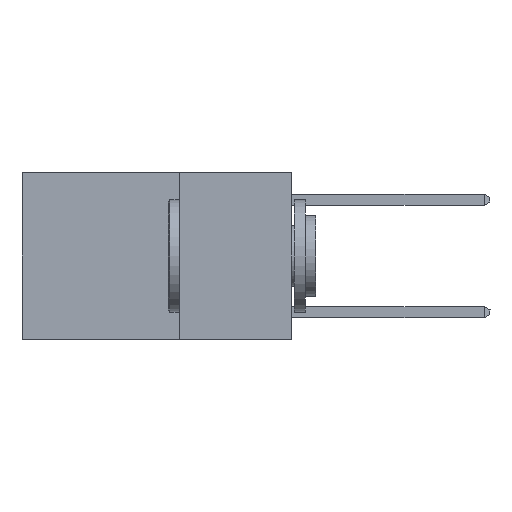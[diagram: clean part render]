
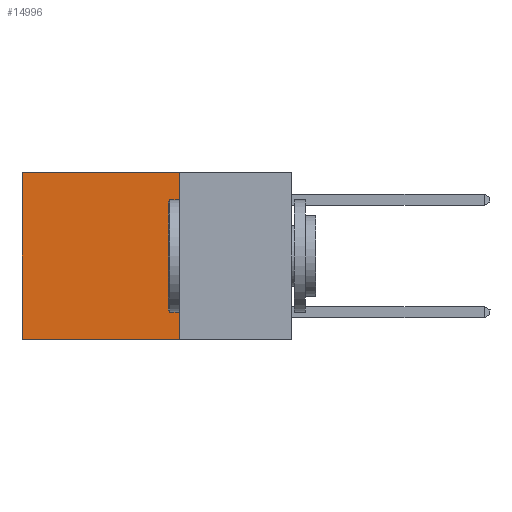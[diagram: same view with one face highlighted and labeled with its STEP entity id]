
A CAD part, left-side view. The second image highlights one B-rep face of the part: STEP entity #14996.
In plain terms, the highlighted planar face has unit normal (-1, 0, 0).
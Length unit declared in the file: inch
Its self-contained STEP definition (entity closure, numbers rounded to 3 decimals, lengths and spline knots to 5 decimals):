
#181 = AXIS2_PLACEMENT_3D ( 'NONE', #5114, #21425, #7490 ) ;
#1319 = EDGE_LOOP ( 'NONE', ( #19151, #2200, #12955, #26617 ) ) ;
#2108 = DIRECTION ( 'NONE',  ( 0., 0., -1. ) ) ;
#2200 = ORIENTED_EDGE ( 'NONE', *, *, #19887, .F. ) ;
#2207 = VECTOR ( 'NONE', #11178, 39.37008 ) ;
#2541 = VERTEX_POINT ( 'NONE', #19791 ) ;
#3071 = VERTEX_POINT ( 'NONE', #17153 ) ;
#5114 = CARTESIAN_POINT ( 'NONE',  ( 0.2625, 0.25, 0. ) ) ;
#6052 = CARTESIAN_POINT ( 'NONE',  ( 0.2625, 0.25, -0.37 ) ) ;
#7490 = DIRECTION ( 'NONE',  ( 0., 0., -1. ) ) ;
#9042 = EDGE_CURVE ( 'NONE', #3071, #2541, #26796, .T. ) ;
#9357 = EDGE_CURVE ( 'NONE', #2541, #21891, #18449, .T. ) ;
#10649 = DIRECTION ( 'NONE',  ( 0., 1., 0. ) ) ;
#11178 = DIRECTION ( 'NONE',  ( 0., 1., 0. ) ) ;
#12040 = LINE ( 'NONE', #29497, #29207 ) ;
#12274 = CARTESIAN_POINT ( 'NONE',  ( 0.2625, 0.6, 0. ) ) ;
#12849 = VERTEX_POINT ( 'NONE', #6052 ) ;
#12955 = ORIENTED_EDGE ( 'NONE', *, *, #15493, .F. ) ;
#12991 = VECTOR ( 'NONE', #14617, 39.37008 ) ;
#14617 = DIRECTION ( 'NONE',  ( 0., 0., -1. ) ) ;
#14996 = ADVANCED_FACE ( 'NONE', ( #18600 ), #27887, .F. ) ;
#15493 = EDGE_CURVE ( 'NONE', #3071, #12849, #12040, .T. ) ;
#17153 = CARTESIAN_POINT ( 'NONE',  ( 0.2625, 0.25, 0. ) ) ;
#18449 = LINE ( 'NONE', #12274, #12991 ) ;
#18600 = FACE_OUTER_BOUND ( 'NONE', #1319, .T. ) ;
#19151 = ORIENTED_EDGE ( 'NONE', *, *, #9357, .T. ) ;
#19791 = CARTESIAN_POINT ( 'NONE',  ( 0.2625, 0.6, 0. ) ) ;
#19859 = VECTOR ( 'NONE', #10649, 39.37008 ) ;
#19887 = EDGE_CURVE ( 'NONE', #12849, #21891, #20584, .T. ) ;
#20163 = CARTESIAN_POINT ( 'NONE',  ( 0.2625, 0.6, -0.37 ) ) ;
#20515 = CARTESIAN_POINT ( 'NONE',  ( 0.2625, 0.25, 0. ) ) ;
#20584 = LINE ( 'NONE', #26527, #19859 ) ;
#21425 = DIRECTION ( 'NONE',  ( 1., 0., 0. ) ) ;
#21891 = VERTEX_POINT ( 'NONE', #20163 ) ;
#26527 = CARTESIAN_POINT ( 'NONE',  ( 0.2625, 0.25, -0.37 ) ) ;
#26617 = ORIENTED_EDGE ( 'NONE', *, *, #9042, .T. ) ;
#26796 = LINE ( 'NONE', #20515, #2207 ) ;
#27887 = PLANE ( 'NONE',  #181 ) ;
#29207 = VECTOR ( 'NONE', #2108, 39.37008 ) ;
#29497 = CARTESIAN_POINT ( 'NONE',  ( 0.2625, 0.25, 0. ) ) ;
